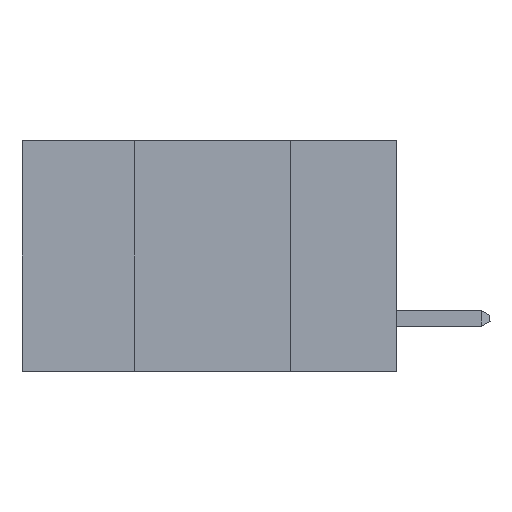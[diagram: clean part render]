
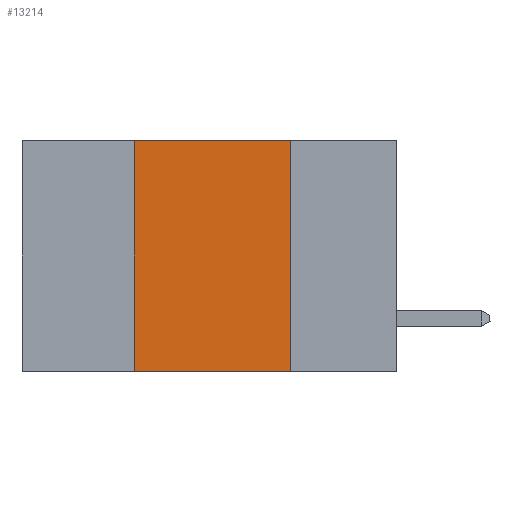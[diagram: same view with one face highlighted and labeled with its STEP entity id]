
A CAD part, left-side view. The second image highlights one B-rep face of the part: STEP entity #13214.
In plain terms, the highlighted planar face has unit normal (-1, 0, 0).
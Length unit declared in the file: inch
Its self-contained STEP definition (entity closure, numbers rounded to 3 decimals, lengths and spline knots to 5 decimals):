
#109 = EDGE_CURVE ( 'NONE', #10729, #1324, #6806, .T. ) ;
#139 = CARTESIAN_POINT ( 'NONE',  ( 0., 0.17, -0.37 ) ) ;
#409 = ORIENTED_EDGE ( 'NONE', *, *, #1708, .F. ) ;
#926 = EDGE_CURVE ( 'NONE', #10729, #1106, #10046, .T. ) ;
#1106 = VERTEX_POINT ( 'NONE', #1497 ) ;
#1324 = VERTEX_POINT ( 'NONE', #139 ) ;
#1336 = EDGE_CURVE ( 'NONE', #1106, #5840, #2011, .T. ) ;
#1497 = CARTESIAN_POINT ( 'NONE',  ( 0., 0.42, 0. ) ) ;
#1708 = EDGE_CURVE ( 'NONE', #5840, #1324, #2733, .T. ) ;
#2001 = CARTESIAN_POINT ( 'NONE',  ( 0., 0.6, -0.37 ) ) ;
#2011 = LINE ( 'NONE', #13382, #7448 ) ;
#2145 = CARTESIAN_POINT ( 'NONE',  ( 0., 0.42, -0.37 ) ) ;
#2421 = PLANE ( 'NONE',  #9054 ) ;
#2468 = DIRECTION ( 'NONE',  ( 1., 0., 0. ) ) ;
#2733 = LINE ( 'NONE', #9613, #8487 ) ;
#2986 = VECTOR ( 'NONE', #3464, 39.37008 ) ;
#3077 = FACE_OUTER_BOUND ( 'NONE', #8080, .T. ) ;
#3464 = DIRECTION ( 'NONE',  ( 0., -1., 0. ) ) ;
#3651 = CARTESIAN_POINT ( 'NONE',  ( 0., 0.6, 0. ) ) ;
#4183 = DIRECTION ( 'NONE',  ( 0., -1., 0. ) ) ;
#4979 = ORIENTED_EDGE ( 'NONE', *, *, #1336, .F. ) ;
#5840 = VERTEX_POINT ( 'NONE', #9876 ) ;
#6806 = LINE ( 'NONE', #2001, #2986 ) ;
#7448 = VECTOR ( 'NONE', #4183, 39.37008 ) ;
#7841 = CARTESIAN_POINT ( 'NONE',  ( 0., 0.42, 0. ) ) ;
#8080 = EDGE_LOOP ( 'NONE', ( #409, #4979, #12366, #13936 ) ) ;
#8487 = VECTOR ( 'NONE', #13354, 39.37008 ) ;
#8519 = DIRECTION ( 'NONE',  ( 0., 0., 1. ) ) ;
#9054 = AXIS2_PLACEMENT_3D ( 'NONE', #3651, #2468, #10450 ) ;
#9613 = CARTESIAN_POINT ( 'NONE',  ( 0., 0.17, 0. ) ) ;
#9676 = VECTOR ( 'NONE', #8519, 39.37008 ) ;
#9876 = CARTESIAN_POINT ( 'NONE',  ( 0., 0.17, 0. ) ) ;
#10046 = LINE ( 'NONE', #7841, #9676 ) ;
#10450 = DIRECTION ( 'NONE',  ( 0., 0., -1. ) ) ;
#10729 = VERTEX_POINT ( 'NONE', #2145 ) ;
#12366 = ORIENTED_EDGE ( 'NONE', *, *, #926, .F. ) ;
#13214 = ADVANCED_FACE ( 'NONE', ( #3077 ), #2421, .F. ) ;
#13354 = DIRECTION ( 'NONE',  ( 0., 0., -1. ) ) ;
#13382 = CARTESIAN_POINT ( 'NONE',  ( 0., 0.6, 0. ) ) ;
#13936 = ORIENTED_EDGE ( 'NONE', *, *, #109, .T. ) ;
